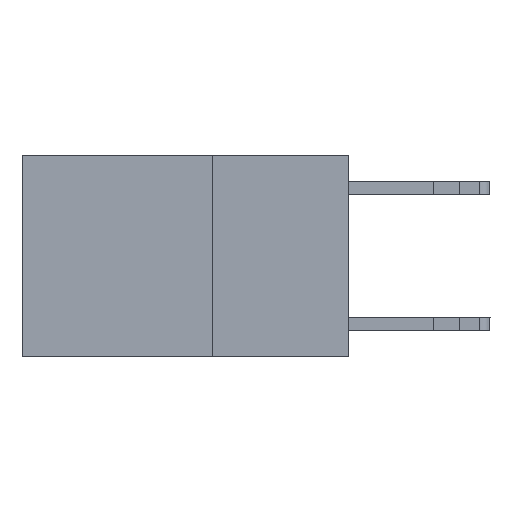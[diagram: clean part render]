
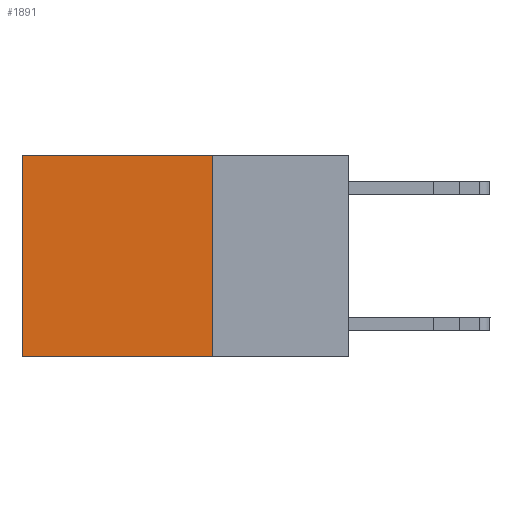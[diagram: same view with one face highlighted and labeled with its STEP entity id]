
A CAD part, left-side view. The second image highlights one B-rep face of the part: STEP entity #1891.
In plain terms, the highlighted planar face has unit normal (-1, 0, 0).
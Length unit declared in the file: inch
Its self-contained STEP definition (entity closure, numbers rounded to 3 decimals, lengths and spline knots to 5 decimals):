
#160 = DIRECTION ( 'NONE',  ( 0., 0., -1. ) ) ;
#279 = DIRECTION ( 'NONE',  ( 0., 0., -1. ) ) ;
#998 = CARTESIAN_POINT ( 'NONE',  ( 0.2625, 0.25, 0. ) ) ;
#1236 = FACE_OUTER_BOUND ( 'NONE', #16647, .T. ) ;
#1891 = ADVANCED_FACE ( 'NONE', ( #1236 ), #21747, .F. ) ;
#2194 = EDGE_CURVE ( 'NONE', #10198, #25128, #16034, .T. ) ;
#2379 = ORIENTED_EDGE ( 'NONE', *, *, #5852, .T. ) ;
#3097 = DIRECTION ( 'NONE',  ( 0., 1., 0. ) ) ;
#3563 = AXIS2_PLACEMENT_3D ( 'NONE', #23924, #13213, #279 ) ;
#3608 = VECTOR ( 'NONE', #160, 39.37008 ) ;
#4104 = VECTOR ( 'NONE', #17061, 39.37008 ) ;
#5852 = EDGE_CURVE ( 'NONE', #11220, #25128, #15529, .T. ) ;
#6773 = LINE ( 'NONE', #998, #23247 ) ;
#8380 = CARTESIAN_POINT ( 'NONE',  ( 0.2625, 0.6, 0. ) ) ;
#9717 = CARTESIAN_POINT ( 'NONE',  ( 0.2625, 0.25, -0.37 ) ) ;
#10013 = LINE ( 'NONE', #17403, #3608 ) ;
#10198 = VERTEX_POINT ( 'NONE', #9717 ) ;
#11220 = VERTEX_POINT ( 'NONE', #8380 ) ;
#12633 = ORIENTED_EDGE ( 'NONE', *, *, #13293, .F. ) ;
#13213 = DIRECTION ( 'NONE',  ( 1., 0., 0. ) ) ;
#13293 = EDGE_CURVE ( 'NONE', #20276, #10198, #10013, .T. ) ;
#13800 = ORIENTED_EDGE ( 'NONE', *, *, #18005, .T. ) ;
#15529 = LINE ( 'NONE', #27787, #4104 ) ;
#16034 = LINE ( 'NONE', #18347, #26831 ) ;
#16647 = EDGE_LOOP ( 'NONE', ( #2379, #25880, #12633, #13800 ) ) ;
#17061 = DIRECTION ( 'NONE',  ( 0., 0., -1. ) ) ;
#17403 = CARTESIAN_POINT ( 'NONE',  ( 0.2625, 0.25, 0. ) ) ;
#17541 = CARTESIAN_POINT ( 'NONE',  ( 0.2625, 0.6, -0.37 ) ) ;
#18005 = EDGE_CURVE ( 'NONE', #20276, #11220, #6773, .T. ) ;
#18347 = CARTESIAN_POINT ( 'NONE',  ( 0.2625, 0.25, -0.37 ) ) ;
#20276 = VERTEX_POINT ( 'NONE', #27450 ) ;
#20505 = DIRECTION ( 'NONE',  ( 0., 1., 0. ) ) ;
#21747 = PLANE ( 'NONE',  #3563 ) ;
#23247 = VECTOR ( 'NONE', #3097, 39.37008 ) ;
#23924 = CARTESIAN_POINT ( 'NONE',  ( 0.2625, 0.25, 0. ) ) ;
#25128 = VERTEX_POINT ( 'NONE', #17541 ) ;
#25880 = ORIENTED_EDGE ( 'NONE', *, *, #2194, .F. ) ;
#26831 = VECTOR ( 'NONE', #20505, 39.37008 ) ;
#27450 = CARTESIAN_POINT ( 'NONE',  ( 0.2625, 0.25, 0. ) ) ;
#27787 = CARTESIAN_POINT ( 'NONE',  ( 0.2625, 0.6, 0. ) ) ;
